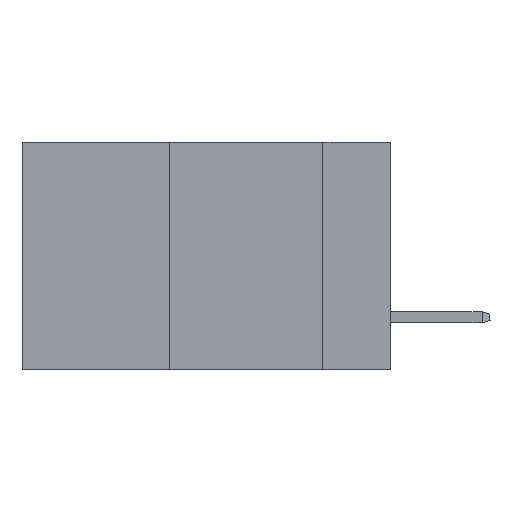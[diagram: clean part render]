
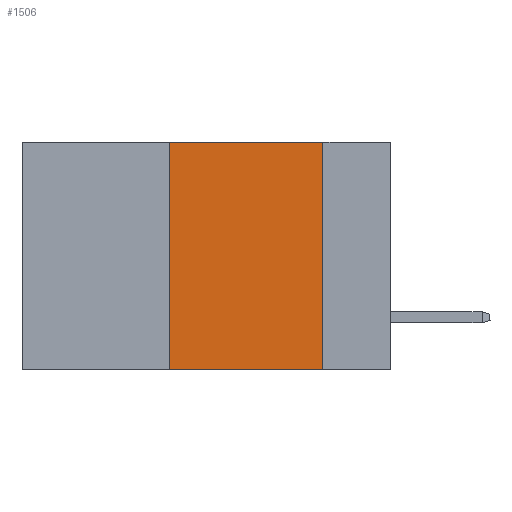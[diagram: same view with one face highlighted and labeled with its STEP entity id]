
A CAD part, left-side view. The second image highlights one B-rep face of the part: STEP entity #1506.
In plain terms, the highlighted planar face has unit normal (-1, 0, 0).
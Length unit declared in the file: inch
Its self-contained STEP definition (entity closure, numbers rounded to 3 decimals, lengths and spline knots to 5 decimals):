
#282 = CARTESIAN_POINT ( 'NONE',  ( 0., 0.6, 0. ) ) ;
#1154 = VERTEX_POINT ( 'NONE', #19752 ) ;
#1497 = FACE_OUTER_BOUND ( 'NONE', #2314, .T. ) ;
#1506 = ADVANCED_FACE ( 'NONE', ( #1497 ), #19159, .F. ) ;
#1635 = VERTEX_POINT ( 'NONE', #3155 ) ;
#1833 = CARTESIAN_POINT ( 'NONE',  ( 0., 0.36, 0. ) ) ;
#1901 = ORIENTED_EDGE ( 'NONE', *, *, #17387, .F. ) ;
#2229 = VERTEX_POINT ( 'NONE', #13272 ) ;
#2314 = EDGE_LOOP ( 'NONE', ( #1901, #10602, #21343, #18313 ) ) ;
#3155 = CARTESIAN_POINT ( 'NONE',  ( 0., 0.36, 0. ) ) ;
#3595 = CARTESIAN_POINT ( 'NONE',  ( 0., 0.6, -0.37 ) ) ;
#4271 = VECTOR ( 'NONE', #17319, 39.37008 ) ;
#5233 = VECTOR ( 'NONE', #15987, 39.37008 ) ;
#6019 = LINE ( 'NONE', #1833, #14792 ) ;
#6988 = DIRECTION ( 'NONE',  ( 0., 0., 1. ) ) ;
#7778 = DIRECTION ( 'NONE',  ( 0., 0., -1. ) ) ;
#8591 = DIRECTION ( 'NONE',  ( 0., 0., -1. ) ) ;
#10602 = ORIENTED_EDGE ( 'NONE', *, *, #11260, .F. ) ;
#11239 = CARTESIAN_POINT ( 'NONE',  ( 0., 0.11, 0. ) ) ;
#11260 = EDGE_CURVE ( 'NONE', #1635, #1154, #14553, .T. ) ;
#12023 = CARTESIAN_POINT ( 'NONE',  ( 0., 0.6, 0. ) ) ;
#12752 = CARTESIAN_POINT ( 'NONE',  ( 0., 0.11, -0.37 ) ) ;
#13272 = CARTESIAN_POINT ( 'NONE',  ( 0., 0.36, -0.37 ) ) ;
#14553 = LINE ( 'NONE', #282, #5233 ) ;
#14792 = VECTOR ( 'NONE', #6988, 39.37008 ) ;
#15987 = DIRECTION ( 'NONE',  ( 0., -1., 0. ) ) ;
#17309 = VERTEX_POINT ( 'NONE', #12752 ) ;
#17319 = DIRECTION ( 'NONE',  ( 0., -1., 0. ) ) ;
#17350 = DIRECTION ( 'NONE',  ( 1., 0., 0. ) ) ;
#17387 = EDGE_CURVE ( 'NONE', #1154, #17309, #21566, .T. ) ;
#17627 = AXIS2_PLACEMENT_3D ( 'NONE', #12023, #17350, #8591 ) ;
#18243 = EDGE_CURVE ( 'NONE', #2229, #1635, #6019, .T. ) ;
#18313 = ORIENTED_EDGE ( 'NONE', *, *, #21326, .T. ) ;
#19159 = PLANE ( 'NONE',  #17627 ) ;
#19752 = CARTESIAN_POINT ( 'NONE',  ( 0., 0.11, 0. ) ) ;
#20081 = LINE ( 'NONE', #3595, #4271 ) ;
#21034 = VECTOR ( 'NONE', #7778, 39.37008 ) ;
#21326 = EDGE_CURVE ( 'NONE', #2229, #17309, #20081, .T. ) ;
#21343 = ORIENTED_EDGE ( 'NONE', *, *, #18243, .F. ) ;
#21566 = LINE ( 'NONE', #11239, #21034 ) ;
